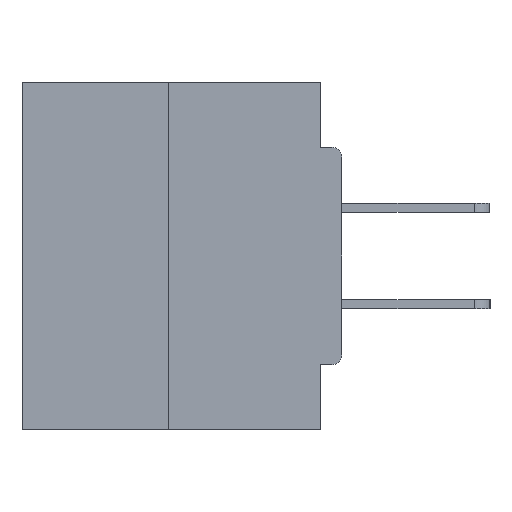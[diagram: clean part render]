
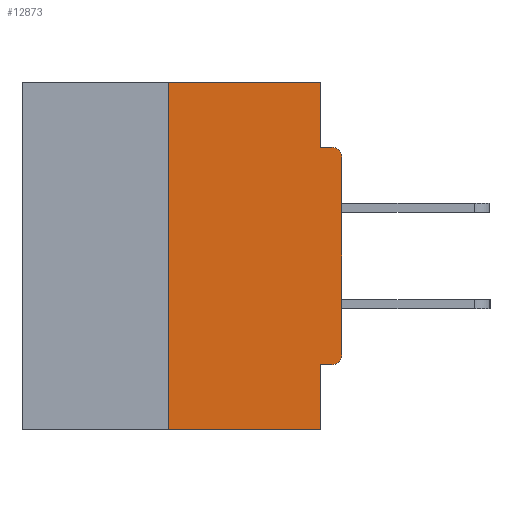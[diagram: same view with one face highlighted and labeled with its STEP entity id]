
A CAD part, left-side view. The second image highlights one B-rep face of the part: STEP entity #12873.
In plain terms, the highlighted planar face has unit normal (-1, 0, 0).
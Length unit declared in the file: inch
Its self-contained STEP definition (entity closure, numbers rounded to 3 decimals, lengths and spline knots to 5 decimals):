
#127 = VERTEX_POINT ( 'NONE', #42335 ) ;
#343 = VERTEX_POINT ( 'NONE', #20087 ) ;
#443 = ORIENTED_EDGE ( 'NONE', *, *, #20817, .F. ) ;
#484 = LINE ( 'NONE', #24435, #39362 ) ;
#589 = CARTESIAN_POINT ( 'NONE',  ( 0., 0.031, 0. ) ) ;
#937 = DIRECTION ( 'NONE',  ( 0., 0., -1. ) ) ;
#1571 = CARTESIAN_POINT ( 'NONE',  ( 0., 0., -0.0935 ) ) ;
#1871 = DIRECTION ( 'NONE',  ( 0., -1., 0. ) ) ;
#3607 = VECTOR ( 'NONE', #1871, 39.37008 ) ;
#3734 = DIRECTION ( 'NONE',  ( 0., 0., 1. ) ) ;
#3742 = PLANE ( 'NONE',  #34345 ) ;
#3744 = VERTEX_POINT ( 'NONE', #16643 ) ;
#3894 = DIRECTION ( 'NONE',  ( 0., 0., -1. ) ) ;
#4901 = CARTESIAN_POINT ( 'NONE',  ( 0., 0.015, -0.1085 ) ) ;
#4984 = CARTESIAN_POINT ( 'NONE',  ( 0., 0.015, -0.3915 ) ) ;
#5059 = DIRECTION ( 'NONE',  ( 0., 0., -1. ) ) ;
#5094 = VECTOR ( 'NONE', #41647, 39.37008 ) ;
#5541 = ORIENTED_EDGE ( 'NONE', *, *, #39701, .F. ) ;
#6723 = CARTESIAN_POINT ( 'NONE',  ( 0., 0., -0.4065 ) ) ;
#8188 = DIRECTION ( 'NONE',  ( 0., -1., 0. ) ) ;
#8921 = LINE ( 'NONE', #589, #5094 ) ;
#10026 = ORIENTED_EDGE ( 'NONE', *, *, #36872, .T. ) ;
#10454 = VECTOR ( 'NONE', #29660, 39.37008 ) ;
#11140 = EDGE_CURVE ( 'NONE', #3744, #14301, #12139, .T. ) ;
#11151 = ORIENTED_EDGE ( 'NONE', *, *, #12440, .F. ) ;
#11936 = CARTESIAN_POINT ( 'NONE',  ( 0., 0.031, -0.4065 ) ) ;
#12139 = LINE ( 'NONE', #23329, #10454 ) ;
#12440 = EDGE_CURVE ( 'NONE', #44718, #16283, #25519, .T. ) ;
#12873 = ADVANCED_FACE ( 'NONE', ( #19553 ), #3742, .F. ) ;
#12898 = CARTESIAN_POINT ( 'NONE',  ( 0., 0.031, -0.0935 ) ) ;
#13191 = VECTOR ( 'NONE', #23714, 39.37008 ) ;
#14301 = VERTEX_POINT ( 'NONE', #26410 ) ;
#16283 = VERTEX_POINT ( 'NONE', #36704 ) ;
#16306 = AXIS2_PLACEMENT_3D ( 'NONE', #4901, #39212, #5059 ) ;
#16643 = CARTESIAN_POINT ( 'NONE',  ( 0., 0., -0.3915 ) ) ;
#16904 = ORIENTED_EDGE ( 'NONE', *, *, #26912, .T. ) ;
#17138 = LINE ( 'NONE', #1571, #3607 ) ;
#17270 = VERTEX_POINT ( 'NONE', #19404 ) ;
#18013 = EDGE_CURVE ( 'NONE', #16283, #38005, #8921, .T. ) ;
#18202 = ORIENTED_EDGE ( 'NONE', *, *, #28906, .F. ) ;
#19404 = CARTESIAN_POINT ( 'NONE',  ( 0., 0.015, -0.4065 ) ) ;
#19553 = FACE_OUTER_BOUND ( 'NONE', #43378, .T. ) ;
#20087 = CARTESIAN_POINT ( 'NONE',  ( 0., 0.015, -0.0935 ) ) ;
#20153 = CARTESIAN_POINT ( 'NONE',  ( 0., 0.25, -0.5 ) ) ;
#20817 = EDGE_CURVE ( 'NONE', #38005, #343, #17138, .T. ) ;
#21390 = VERTEX_POINT ( 'NONE', #20153 ) ;
#21731 = EDGE_CURVE ( 'NONE', #17270, #3744, #40788, .T. ) ;
#23329 = CARTESIAN_POINT ( 'NONE',  ( 0., 0., 0. ) ) ;
#23714 = DIRECTION ( 'NONE',  ( 0., -1., 0. ) ) ;
#24435 = CARTESIAN_POINT ( 'NONE',  ( 0., 0.25, 0. ) ) ;
#24748 = DIRECTION ( 'NONE',  ( 1., 0., 0. ) ) ;
#24855 = VECTOR ( 'NONE', #38132, 39.37008 ) ;
#25420 = EDGE_CURVE ( 'NONE', #21390, #44718, #484, .T. ) ;
#25519 = LINE ( 'NONE', #39558, #44494 ) ;
#25911 = LINE ( 'NONE', #6723, #24855 ) ;
#26410 = CARTESIAN_POINT ( 'NONE',  ( 0., 0., -0.1085 ) ) ;
#26587 = LINE ( 'NONE', #42294, #30954 ) ;
#26909 = ORIENTED_EDGE ( 'NONE', *, *, #25420, .F. ) ;
#26912 = EDGE_CURVE ( 'NONE', #21390, #127, #40700, .T. ) ;
#27285 = VERTEX_POINT ( 'NONE', #11936 ) ;
#28906 = EDGE_CURVE ( 'NONE', #17270, #27285, #25911, .T. ) ;
#29660 = DIRECTION ( 'NONE',  ( 0., 0., 1. ) ) ;
#30954 = VECTOR ( 'NONE', #937, 39.37008 ) ;
#31236 = ORIENTED_EDGE ( 'NONE', *, *, #18013, .F. ) ;
#32943 = DIRECTION ( 'NONE',  ( -1., 0., 0. ) ) ;
#34345 = AXIS2_PLACEMENT_3D ( 'NONE', #38037, #24748, #3894 ) ;
#35349 = ORIENTED_EDGE ( 'NONE', *, *, #11140, .T. ) ;
#36704 = CARTESIAN_POINT ( 'NONE',  ( 0., 0.031, 0. ) ) ;
#36872 = EDGE_CURVE ( 'NONE', #14301, #343, #42660, .T. ) ;
#38005 = VERTEX_POINT ( 'NONE', #12898 ) ;
#38037 = CARTESIAN_POINT ( 'NONE',  ( 0., 0.46, 0. ) ) ;
#38132 = DIRECTION ( 'NONE',  ( 0., 1., 0. ) ) ;
#38671 = AXIS2_PLACEMENT_3D ( 'NONE', #4984, #32943, #39425 ) ;
#39212 = DIRECTION ( 'NONE',  ( -1., 0., 0. ) ) ;
#39362 = VECTOR ( 'NONE', #3734, 39.37008 ) ;
#39425 = DIRECTION ( 'NONE',  ( 0., 0., -1. ) ) ;
#39558 = CARTESIAN_POINT ( 'NONE',  ( 0., 0.46, 0. ) ) ;
#39701 = EDGE_CURVE ( 'NONE', #27285, #127, #26587, .T. ) ;
#40700 = LINE ( 'NONE', #40929, #13191 ) ;
#40788 = CIRCLE ( 'NONE', #38671, 0.015 ) ;
#40929 = CARTESIAN_POINT ( 'NONE',  ( 0., 0.46, -0.5 ) ) ;
#41647 = DIRECTION ( 'NONE',  ( 0., 0., -1. ) ) ;
#42294 = CARTESIAN_POINT ( 'NONE',  ( 0., 0.031, -0.5 ) ) ;
#42335 = CARTESIAN_POINT ( 'NONE',  ( 0., 0.031, -0.5 ) ) ;
#42660 = CIRCLE ( 'NONE', #16306, 0.015 ) ;
#42691 = ORIENTED_EDGE ( 'NONE', *, *, #21731, .T. ) ;
#43121 = CARTESIAN_POINT ( 'NONE',  ( 0., 0.25, 0. ) ) ;
#43378 = EDGE_LOOP ( 'NONE', ( #11151, #26909, #16904, #5541, #18202, #42691, #35349, #10026, #443, #31236 ) ) ;
#44494 = VECTOR ( 'NONE', #8188, 39.37008 ) ;
#44718 = VERTEX_POINT ( 'NONE', #43121 ) ;
